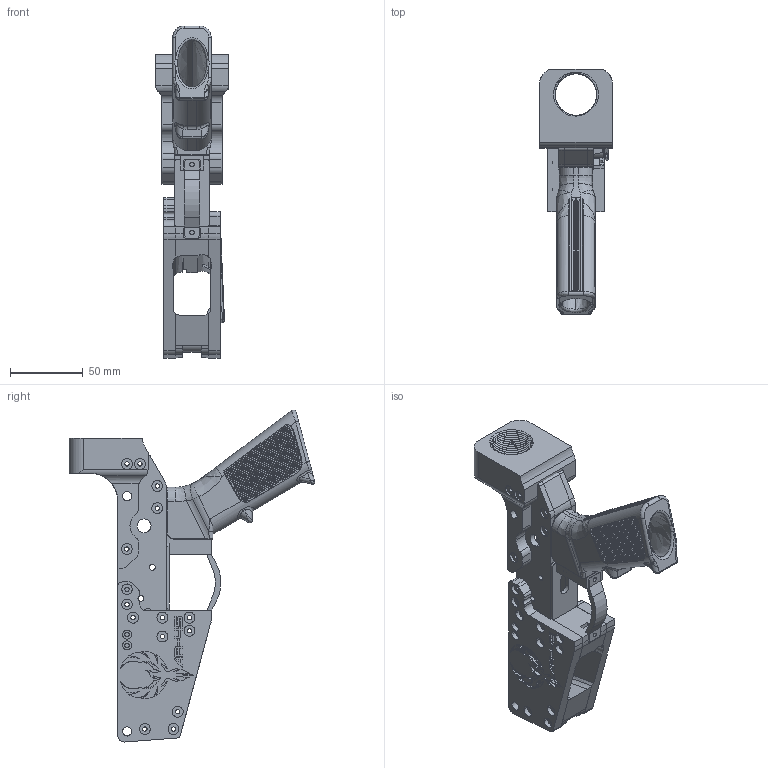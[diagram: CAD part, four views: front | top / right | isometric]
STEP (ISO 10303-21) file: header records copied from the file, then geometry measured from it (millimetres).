
FILE_DESCRIPTION (( 'STEP AP214' ), '1' );
FILE_NAME ('Firebolt_45_Standard.STEP', '2020-12-05T19:00:30', ( '' ), ( '' ), 'SwSTEP 2.0', 'SolidWorks 2020', '' );
FILE_SCHEMA (( 'AUTOMOTIVE_DESIGN' ));
Length unit declared in the file: millimetre
Products named in the file (13): Firebolt_45_Mag_Well_Right; Firebolt_45_Standard; Mag_Release; Firebolt_45_Mag_Well_Left; Firebolt_Side_Right; Firebolt_Fire_Control_Well_Bottom; Firebolt_45_Mag_Well_Front; Firebolt_Pistol_Grip; Firebolt_45_Mag_Well_Rear; Firebolt_Side_Left; Firebolt_Grip_Part; Firebolt_Trigger_Guard; Firebolt_Buffer_Tower
Assembly tree (12 placements, depth 2):
  Firebolt_45_Standard
    Firebolt_Buffer_Tower
    Firebolt_Side_Left
    Firebolt_Side_Right
    Firebolt_Grip_Part
    Firebolt_Pistol_Grip
    Firebolt_Fire_Control_Well_Bottom
    Firebolt_Trigger_Guard
    Firebolt_45_Mag_Well_Rear
    Firebolt_45_Mag_Well_Right
    Firebolt_45_Mag_Well_Left
    Firebolt_45_Mag_Well_Front
    Mag_Release
Bounding box: 50 x 169.01 x 228.64 mm (x, y, z)
Volume: 284776.1 mm3; surface area: 125328.6 mm2
Topology: 12 solids, 12 shells, 8071 faces, 17831 edges, 11321 vertices
Faces by surface type: plane 7304, cylinder 537, bspline 204, cone 20, torus 6
Entity records: 258814 total; most frequent: CARTESIAN_POINT 87376, ORIENTED_EDGE 35642, DIRECTION 30799, EDGE_CURVE 17821, VECTOR 13185, LINE 13185, VERTEX_POINT 11321, EDGE_LOOP 9804
